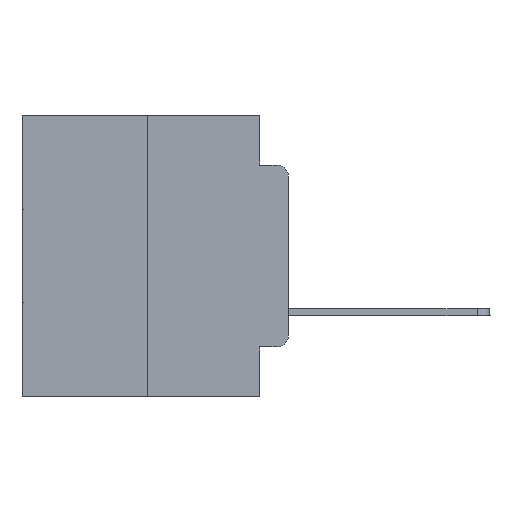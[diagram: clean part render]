
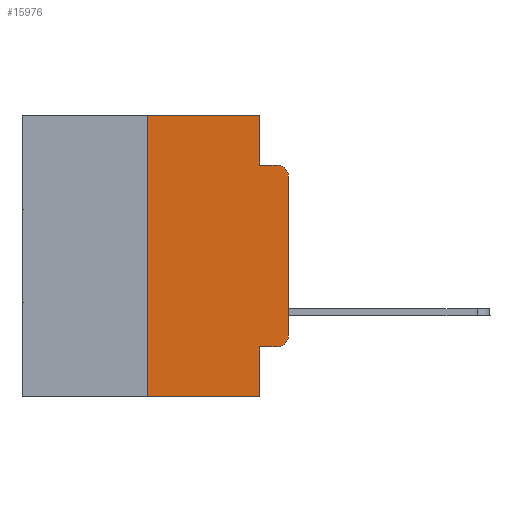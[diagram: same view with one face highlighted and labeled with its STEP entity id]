
A CAD part, left-side view. The second image highlights one B-rep face of the part: STEP entity #15976.
In plain terms, the highlighted planar face has unit normal (-1, 0, 0).
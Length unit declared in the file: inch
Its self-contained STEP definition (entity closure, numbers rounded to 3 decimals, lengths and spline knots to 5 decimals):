
#352 = VERTEX_POINT ( 'NONE', #21359 ) ;
#1309 = CARTESIAN_POINT ( 'NONE',  ( 0., 0.051, 0. ) ) ;
#2334 = EDGE_CURVE ( 'NONE', #11791, #6258, #12674, .T. ) ;
#2406 = VECTOR ( 'NONE', #12719, 39.37008 ) ;
#3013 = EDGE_CURVE ( 'NONE', #24914, #16941, #21977, .T. ) ;
#3373 = ORIENTED_EDGE ( 'NONE', *, *, #26135, .F. ) ;
#3657 = DIRECTION ( 'NONE',  ( 0., -1., 0. ) ) ;
#5009 = CARTESIAN_POINT ( 'NONE',  ( 0., 0.25, -0.5 ) ) ;
#5425 = CARTESIAN_POINT ( 'NONE',  ( 0., 0.051, -0.0885 ) ) ;
#6258 = VERTEX_POINT ( 'NONE', #12847 ) ;
#6401 = CARTESIAN_POINT ( 'NONE',  ( 0., 0.051, 0. ) ) ;
#7395 = ORIENTED_EDGE ( 'NONE', *, *, #28050, .F. ) ;
#8567 = DIRECTION ( 'NONE',  ( 0., 0., -1. ) ) ;
#8786 = ORIENTED_EDGE ( 'NONE', *, *, #3013, .F. ) ;
#9015 = EDGE_CURVE ( 'NONE', #352, #11791, #17618, .T. ) ;
#9098 = VECTOR ( 'NONE', #14888, 39.37008 ) ;
#9500 = DIRECTION ( 'NONE',  ( 0., 0., 1. ) ) ;
#9514 = ORIENTED_EDGE ( 'NONE', *, *, #16583, .T. ) ;
#9658 = LINE ( 'NONE', #19207, #2406 ) ;
#11125 = EDGE_LOOP ( 'NONE', ( #24753, #28484, #26359, #8786, #3373, #7395, #28496, #12153, #9514, #16585 ) ) ;
#11575 = DIRECTION ( 'NONE',  ( 0., 0., -1. ) ) ;
#11791 = VERTEX_POINT ( 'NONE', #14182 ) ;
#12153 = ORIENTED_EDGE ( 'NONE', *, *, #20124, .F. ) ;
#12674 = CIRCLE ( 'NONE', #18903, 0.02 ) ;
#12719 = DIRECTION ( 'NONE',  ( 0., -1., 0. ) ) ;
#12815 = VECTOR ( 'NONE', #20887, 39.37008 ) ;
#12847 = CARTESIAN_POINT ( 'NONE',  ( 0., 0.02, -0.0885 ) ) ;
#12871 = CARTESIAN_POINT ( 'NONE',  ( 0., 0.051, -0.4115 ) ) ;
#12939 = VECTOR ( 'NONE', #21896, 39.37008 ) ;
#13247 = CARTESIAN_POINT ( 'NONE',  ( 0., 0.02, -0.3915 ) ) ;
#13399 = VERTEX_POINT ( 'NONE', #5009 ) ;
#13664 = DIRECTION ( 'NONE',  ( 0., 0., -1. ) ) ;
#13806 = DIRECTION ( 'NONE',  ( -1., 0., 0. ) ) ;
#14182 = CARTESIAN_POINT ( 'NONE',  ( 0., 0., -0.1085 ) ) ;
#14207 = VECTOR ( 'NONE', #3657, 39.37008 ) ;
#14422 = VERTEX_POINT ( 'NONE', #14848 ) ;
#14501 = EDGE_CURVE ( 'NONE', #16941, #6258, #15660, .T. ) ;
#14561 = CARTESIAN_POINT ( 'NONE',  ( 0., 0.02, -0.4115 ) ) ;
#14848 = CARTESIAN_POINT ( 'NONE',  ( 0., 0.051, -0.5 ) ) ;
#14852 = CARTESIAN_POINT ( 'NONE',  ( 0., 0.473, 0. ) ) ;
#14888 = DIRECTION ( 'NONE',  ( 0., -1., 0. ) ) ;
#14967 = CARTESIAN_POINT ( 'NONE',  ( 0., 0.051, 0. ) ) ;
#15192 = VECTOR ( 'NONE', #9500, 39.37008 ) ;
#15660 = LINE ( 'NONE', #18163, #27756 ) ;
#15865 = DIRECTION ( 'NONE',  ( 0., -1., 0. ) ) ;
#15976 = ADVANCED_FACE ( 'NONE', ( #21847 ), #25706, .F. ) ;
#16061 = VECTOR ( 'NONE', #21651, 39.37008 ) ;
#16346 = VERTEX_POINT ( 'NONE', #14561 ) ;
#16583 = EDGE_CURVE ( 'NONE', #20789, #16346, #9658, .T. ) ;
#16585 = ORIENTED_EDGE ( 'NONE', *, *, #24060, .T. ) ;
#16746 = AXIS2_PLACEMENT_3D ( 'NONE', #13247, #13806, #11575 ) ;
#16941 = VERTEX_POINT ( 'NONE', #5425 ) ;
#17561 = CARTESIAN_POINT ( 'NONE',  ( 0., 0.473, 0. ) ) ;
#17618 = LINE ( 'NONE', #24203, #12815 ) ;
#18163 = CARTESIAN_POINT ( 'NONE',  ( 0., 0.051, -0.0885 ) ) ;
#18696 = CARTESIAN_POINT ( 'NONE',  ( 0., 0.25, 0. ) ) ;
#18903 = AXIS2_PLACEMENT_3D ( 'NONE', #26875, #24746, #13664 ) ;
#19156 = CARTESIAN_POINT ( 'NONE',  ( 0., 0.473, -0.5 ) ) ;
#19207 = CARTESIAN_POINT ( 'NONE',  ( 0., 0.051, -0.4115 ) ) ;
#19823 = DIRECTION ( 'NONE',  ( 1., 0., 0. ) ) ;
#20124 = EDGE_CURVE ( 'NONE', #20789, #14422, #20897, .T. ) ;
#20365 = LINE ( 'NONE', #18696, #15192 ) ;
#20621 = EDGE_CURVE ( 'NONE', #13399, #14422, #20948, .T. ) ;
#20789 = VERTEX_POINT ( 'NONE', #12871 ) ;
#20887 = DIRECTION ( 'NONE',  ( 0., 0., 1. ) ) ;
#20897 = LINE ( 'NONE', #6401, #12939 ) ;
#20948 = LINE ( 'NONE', #19156, #9098 ) ;
#21359 = CARTESIAN_POINT ( 'NONE',  ( 0., 0., -0.3915 ) ) ;
#21651 = DIRECTION ( 'NONE',  ( 0., 0., -1. ) ) ;
#21847 = FACE_OUTER_BOUND ( 'NONE', #11125, .T. ) ;
#21896 = DIRECTION ( 'NONE',  ( 0., 0., -1. ) ) ;
#21977 = LINE ( 'NONE', #14967, #16061 ) ;
#24060 = EDGE_CURVE ( 'NONE', #16346, #352, #24689, .T. ) ;
#24203 = CARTESIAN_POINT ( 'NONE',  ( 0., 0., 0. ) ) ;
#24260 = CARTESIAN_POINT ( 'NONE',  ( 0., 0.25, 0. ) ) ;
#24689 = CIRCLE ( 'NONE', #16746, 0.02 ) ;
#24746 = DIRECTION ( 'NONE',  ( -1., 0., 0. ) ) ;
#24753 = ORIENTED_EDGE ( 'NONE', *, *, #9015, .T. ) ;
#24914 = VERTEX_POINT ( 'NONE', #1309 ) ;
#25118 = AXIS2_PLACEMENT_3D ( 'NONE', #17561, #19823, #8567 ) ;
#25706 = PLANE ( 'NONE',  #25118 ) ;
#26135 = EDGE_CURVE ( 'NONE', #27133, #24914, #26634, .T. ) ;
#26359 = ORIENTED_EDGE ( 'NONE', *, *, #14501, .F. ) ;
#26634 = LINE ( 'NONE', #14852, #14207 ) ;
#26875 = CARTESIAN_POINT ( 'NONE',  ( 0., 0.02, -0.1085 ) ) ;
#27133 = VERTEX_POINT ( 'NONE', #24260 ) ;
#27756 = VECTOR ( 'NONE', #15865, 39.37008 ) ;
#28050 = EDGE_CURVE ( 'NONE', #13399, #27133, #20365, .T. ) ;
#28484 = ORIENTED_EDGE ( 'NONE', *, *, #2334, .T. ) ;
#28496 = ORIENTED_EDGE ( 'NONE', *, *, #20621, .T. ) ;
